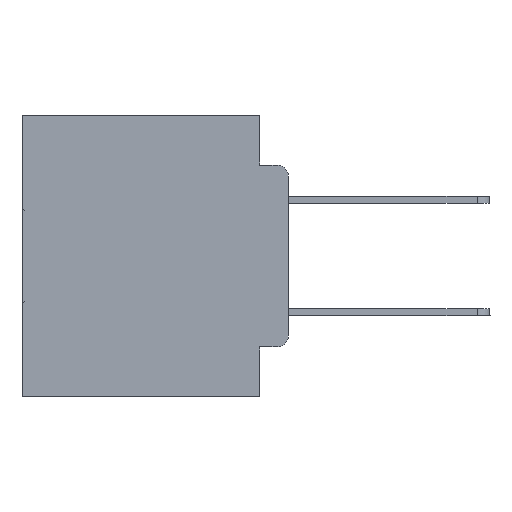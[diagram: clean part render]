
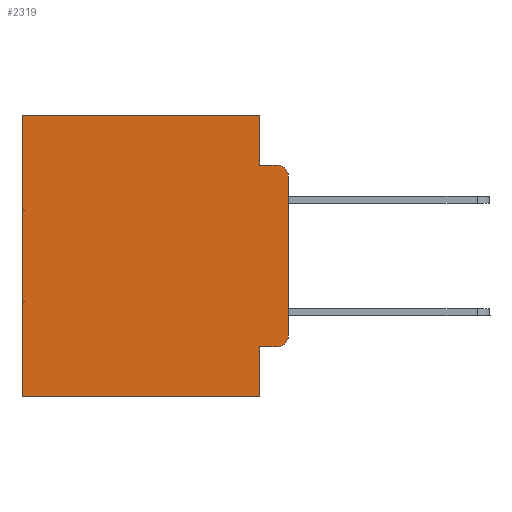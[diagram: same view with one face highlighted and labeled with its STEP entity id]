
A CAD part, left-side view. The second image highlights one B-rep face of the part: STEP entity #2319.
In plain terms, the highlighted planar face has unit normal (-1, 0, 0).
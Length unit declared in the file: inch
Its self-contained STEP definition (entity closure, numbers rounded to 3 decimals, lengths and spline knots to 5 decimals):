
#307 = CARTESIAN_POINT ( 'NONE',  ( 0.298, 0.051, 0. ) ) ;
#643 = EDGE_CURVE ( 'NONE', #32800, #13702, #976, .T. ) ;
#809 = ORIENTED_EDGE ( 'NONE', *, *, #33802, .T. ) ;
#976 = LINE ( 'NONE', #19351, #8278 ) ;
#1681 = DIRECTION ( 'NONE',  ( 0., 0., -1. ) ) ;
#1790 = LINE ( 'NONE', #12427, #28103 ) ;
#1819 = VERTEX_POINT ( 'NONE', #10474 ) ;
#2319 = ADVANCED_FACE ( 'NONE', ( #11592 ), #16400, .F. ) ;
#2441 = EDGE_CURVE ( 'NONE', #31051, #27492, #1790, .T. ) ;
#3338 = CARTESIAN_POINT ( 'NONE',  ( 0.298, 0.051, -0.4115 ) ) ;
#3345 = CARTESIAN_POINT ( 'NONE',  ( 0.298, 0.051, -0.4115 ) ) ;
#3999 = CARTESIAN_POINT ( 'NONE',  ( 0.298, 0.051, -0.5 ) ) ;
#4510 = VERTEX_POINT ( 'NONE', #19243 ) ;
#4567 = DIRECTION ( 'NONE',  ( 0., 1., 0. ) ) ;
#5424 = VECTOR ( 'NONE', #18039, 39.37008 ) ;
#5429 = ORIENTED_EDGE ( 'NONE', *, *, #643, .F. ) ;
#5445 = DIRECTION ( 'NONE',  ( 0., -1., 0. ) ) ;
#6767 = DIRECTION ( 'NONE',  ( 0., 1., 0. ) ) ;
#6928 = CARTESIAN_POINT ( 'NONE',  ( 0.298, 0.051, -0.0885 ) ) ;
#7559 = CARTESIAN_POINT ( 'NONE',  ( 0.298, 0.473, 0. ) ) ;
#7678 = ORIENTED_EDGE ( 'NONE', *, *, #21645, .F. ) ;
#8278 = VECTOR ( 'NONE', #9214, 39.37008 ) ;
#8491 = ORIENTED_EDGE ( 'NONE', *, *, #18298, .T. ) ;
#8668 = DIRECTION ( 'NONE',  ( 1., 0., 0. ) ) ;
#8737 = VERTEX_POINT ( 'NONE', #6928 ) ;
#9214 = DIRECTION ( 'NONE',  ( 0., 0., -1. ) ) ;
#9252 = CARTESIAN_POINT ( 'NONE',  ( 0.298, 0.02, -0.3915 ) ) ;
#9543 = VERTEX_POINT ( 'NONE', #12506 ) ;
#9555 = DIRECTION ( 'NONE',  ( -1., 0., 0. ) ) ;
#9784 = EDGE_CURVE ( 'NONE', #8737, #4510, #31275, .T. ) ;
#10474 = CARTESIAN_POINT ( 'NONE',  ( 0.298, 0.473, -0.5 ) ) ;
#11592 = FACE_OUTER_BOUND ( 'NONE', #16297, .T. ) ;
#12427 = CARTESIAN_POINT ( 'NONE',  ( 0.298, 0., 0. ) ) ;
#12506 = CARTESIAN_POINT ( 'NONE',  ( 0.298, 0.02, -0.4115 ) ) ;
#13141 = LINE ( 'NONE', #28172, #24720 ) ;
#13702 = VERTEX_POINT ( 'NONE', #3999 ) ;
#13800 = LINE ( 'NONE', #3338, #20544 ) ;
#14584 = ORIENTED_EDGE ( 'NONE', *, *, #26093, .T. ) ;
#14710 = ORIENTED_EDGE ( 'NONE', *, *, #9784, .F. ) ;
#16297 = EDGE_LOOP ( 'NONE', ( #7678, #14584, #14710, #30845, #22831, #27412, #26701, #5429, #8491, #809 ) ) ;
#16400 = PLANE ( 'NONE',  #27775 ) ;
#17244 = EDGE_CURVE ( 'NONE', #31051, #8737, #31625, .T. ) ;
#18039 = DIRECTION ( 'NONE',  ( 0., 0., -1. ) ) ;
#18298 = EDGE_CURVE ( 'NONE', #32800, #9543, #13800, .T. ) ;
#18308 = VERTEX_POINT ( 'NONE', #24819 ) ;
#19243 = CARTESIAN_POINT ( 'NONE',  ( 0.298, 0.02, -0.0885 ) ) ;
#19351 = CARTESIAN_POINT ( 'NONE',  ( 0.298, 0.051, 0. ) ) ;
#19516 = CIRCLE ( 'NONE', #29985, 0.02 ) ;
#20544 = VECTOR ( 'NONE', #21696, 39.37008 ) ;
#20602 = VECTOR ( 'NONE', #5445, 39.37008 ) ;
#21601 = DIRECTION ( 'NONE',  ( 0., 0., -1. ) ) ;
#21645 = EDGE_CURVE ( 'NONE', #33553, #18308, #32134, .T. ) ;
#21696 = DIRECTION ( 'NONE',  ( 0., -1., 0. ) ) ;
#21980 = DIRECTION ( 'NONE',  ( 0., 0., -1. ) ) ;
#22812 = CARTESIAN_POINT ( 'NONE',  ( 0.298, 0.051, 0. ) ) ;
#22831 = ORIENTED_EDGE ( 'NONE', *, *, #2441, .T. ) ;
#23573 = CIRCLE ( 'NONE', #32375, 0.02 ) ;
#24016 = EDGE_CURVE ( 'NONE', #27492, #1819, #31655, .T. ) ;
#24046 = DIRECTION ( 'NONE',  ( 0., 0., -1. ) ) ;
#24720 = VECTOR ( 'NONE', #4567, 39.37008 ) ;
#24819 = CARTESIAN_POINT ( 'NONE',  ( 0.298, 0., -0.3915 ) ) ;
#25001 = EDGE_CURVE ( 'NONE', #13702, #1819, #13141, .T. ) ;
#25406 = CARTESIAN_POINT ( 'NONE',  ( 0.298, 0.02, -0.1085 ) ) ;
#26093 = EDGE_CURVE ( 'NONE', #33553, #4510, #23573, .T. ) ;
#26701 = ORIENTED_EDGE ( 'NONE', *, *, #25001, .F. ) ;
#27007 = DIRECTION ( 'NONE',  ( -1., 0., 0. ) ) ;
#27101 = CARTESIAN_POINT ( 'NONE',  ( 0.298, 0., 0. ) ) ;
#27412 = ORIENTED_EDGE ( 'NONE', *, *, #24016, .T. ) ;
#27492 = VERTEX_POINT ( 'NONE', #28075 ) ;
#27775 = AXIS2_PLACEMENT_3D ( 'NONE', #27101, #8668, #30190 ) ;
#28075 = CARTESIAN_POINT ( 'NONE',  ( 0.298, 0.473, 0. ) ) ;
#28103 = VECTOR ( 'NONE', #6767, 39.37008 ) ;
#28172 = CARTESIAN_POINT ( 'NONE',  ( 0.298, 0., -0.5 ) ) ;
#29038 = CARTESIAN_POINT ( 'NONE',  ( 0.298, 0.051, -0.0885 ) ) ;
#29237 = CARTESIAN_POINT ( 'NONE',  ( 0.298, 0., -0.1085 ) ) ;
#29574 = CARTESIAN_POINT ( 'NONE',  ( 0.298, 0., 0. ) ) ;
#29985 = AXIS2_PLACEMENT_3D ( 'NONE', #9252, #27007, #21980 ) ;
#30190 = DIRECTION ( 'NONE',  ( 0., 0., -1. ) ) ;
#30845 = ORIENTED_EDGE ( 'NONE', *, *, #17244, .F. ) ;
#31051 = VERTEX_POINT ( 'NONE', #22812 ) ;
#31275 = LINE ( 'NONE', #29038, #20602 ) ;
#31625 = LINE ( 'NONE', #307, #33174 ) ;
#31655 = LINE ( 'NONE', #7559, #5424 ) ;
#32134 = LINE ( 'NONE', #29574, #33867 ) ;
#32375 = AXIS2_PLACEMENT_3D ( 'NONE', #25406, #9555, #1681 ) ;
#32800 = VERTEX_POINT ( 'NONE', #3345 ) ;
#33174 = VECTOR ( 'NONE', #21601, 39.37008 ) ;
#33553 = VERTEX_POINT ( 'NONE', #29237 ) ;
#33802 = EDGE_CURVE ( 'NONE', #9543, #18308, #19516, .T. ) ;
#33867 = VECTOR ( 'NONE', #24046, 39.37008 ) ;
